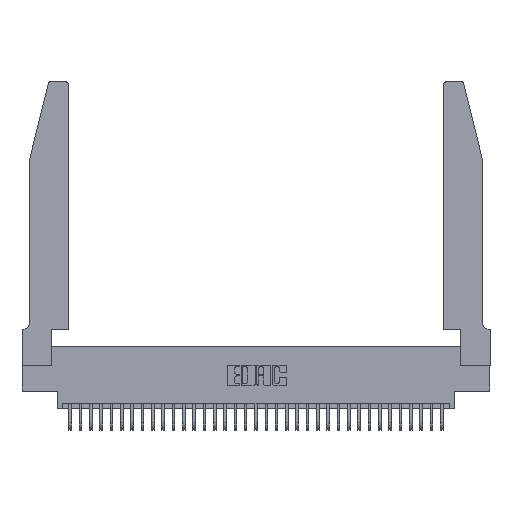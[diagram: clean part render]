
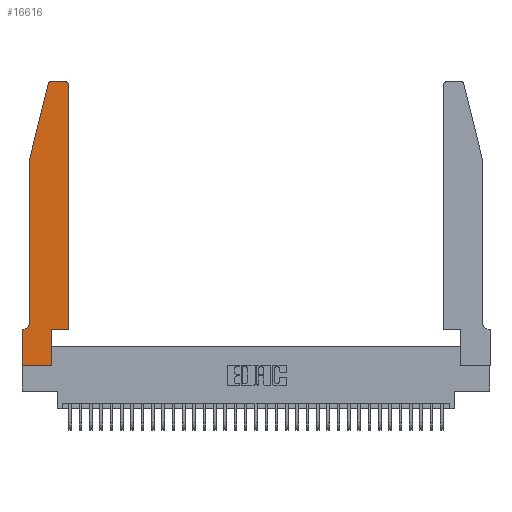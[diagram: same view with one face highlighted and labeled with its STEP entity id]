
A CAD part, top view. The second image highlights one B-rep face of the part: STEP entity #16616.
In plain terms, the highlighted planar face has unit normal (0, 0, 1).
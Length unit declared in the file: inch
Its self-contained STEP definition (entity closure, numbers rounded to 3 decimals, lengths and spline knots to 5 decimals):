
#65 = ORIENTED_EDGE ( 'NONE', *, *, #2224, .T. ) ;
#76 = VERTEX_POINT ( 'NONE', #10745 ) ;
#1164 = CARTESIAN_POINT ( 'NONE',  ( 0.4205, 2.75, 0.37 ) ) ;
#1331 = VERTEX_POINT ( 'NONE', #31870 ) ;
#1661 = VERTEX_POINT ( 'NONE', #2278 ) ;
#2116 = DIRECTION ( 'NONE',  ( -1., 0., 0. ) ) ;
#2174 = VECTOR ( 'NONE', #16784, 39.37008 ) ;
#2224 = EDGE_CURVE ( 'NONE', #10410, #76, #25357, .T. ) ;
#2278 = CARTESIAN_POINT ( 'NONE',  ( 0.2865, 0.35, 0.37 ) ) ;
#2492 = DIRECTION ( 'NONE',  ( 0., 1., 0. ) ) ;
#2646 = CARTESIAN_POINT ( 'NONE',  ( 0.4505, 2.72, 0.37 ) ) ;
#2780 = CARTESIAN_POINT ( 'NONE',  ( 0., 0., 0.37 ) ) ;
#3082 = LINE ( 'NONE', #16886, #2174 ) ;
#3813 = ORIENTED_EDGE ( 'NONE', *, *, #25505, .T. ) ;
#4161 = CARTESIAN_POINT ( 'NONE',  ( 0.0755, 2., 0.37 ) ) ;
#4770 = CARTESIAN_POINT ( 'NONE',  ( 0.0755, 2., 0.37 ) ) ;
#4788 = CARTESIAN_POINT ( 'NONE',  ( 0., 0.35, 0.37 ) ) ;
#5586 = DIRECTION ( 'NONE',  ( 1., 0., 0. ) ) ;
#5776 = EDGE_CURVE ( 'NONE', #76, #24722, #29661, .T. ) ;
#6999 = DIRECTION ( 'NONE',  ( -0.239, -0.971, 0. ) ) ;
#7488 = VERTEX_POINT ( 'NONE', #25301 ) ;
#8725 = EDGE_CURVE ( 'NONE', #26571, #1661, #8899, .T. ) ;
#8899 = LINE ( 'NONE', #36023, #22948 ) ;
#9705 = DIRECTION ( 'NONE',  ( 0., 1., 0. ) ) ;
#10109 = EDGE_CURVE ( 'NONE', #1661, #16941, #3082, .T. ) ;
#10286 = AXIS2_PLACEMENT_3D ( 'NONE', #35688, #19027, #2116 ) ;
#10410 = VERTEX_POINT ( 'NONE', #1164 ) ;
#10497 = DIRECTION ( 'NONE',  ( 0., 0., 1. ) ) ;
#10745 = CARTESIAN_POINT ( 'NONE',  ( 0.284, 2.75, 0.37 ) ) ;
#12527 = LINE ( 'NONE', #4770, #32239 ) ;
#12644 = ORIENTED_EDGE ( 'NONE', *, *, #10109, .T. ) ;
#13102 = DIRECTION ( 'NONE',  ( 0., -1., 0. ) ) ;
#13213 = ORIENTED_EDGE ( 'NONE', *, *, #24683, .T. ) ;
#13678 = CARTESIAN_POINT ( 'NONE',  ( 0.4205, 2.72, 0.37 ) ) ;
#14439 = AXIS2_PLACEMENT_3D ( 'NONE', #15244, #34764, #18112 ) ;
#15244 = CARTESIAN_POINT ( 'NONE',  ( 0.284, 2.72, 0.37 ) ) ;
#16072 = DIRECTION ( 'NONE',  ( -1., 0., 0. ) ) ;
#16124 = CARTESIAN_POINT ( 'NONE',  ( 0.0755, 0.35, 0.37 ) ) ;
#16552 = DIRECTION ( 'NONE',  ( 1., 0., 0. ) ) ;
#16616 = ADVANCED_FACE ( 'NONE', ( #25283 ), #27270, .T. ) ;
#16645 = VECTOR ( 'NONE', #5586, 39.37008 ) ;
#16696 = EDGE_CURVE ( 'NONE', #31564, #10410, #30940, .T. ) ;
#16701 = VERTEX_POINT ( 'NONE', #22013 ) ;
#16784 = DIRECTION ( 'NONE',  ( 1., 0., 0. ) ) ;
#16886 = CARTESIAN_POINT ( 'NONE',  ( 0.4505, 0.35, 0.37 ) ) ;
#16941 = VERTEX_POINT ( 'NONE', #28585 ) ;
#17128 = EDGE_CURVE ( 'NONE', #16941, #31564, #18732, .T. ) ;
#17242 = EDGE_CURVE ( 'NONE', #33891, #1331, #28287, .T. ) ;
#17891 = EDGE_CURVE ( 'NONE', #34405, #33891, #22990, .T. ) ;
#17976 = VECTOR ( 'NONE', #16072, 39.37008 ) ;
#18112 = DIRECTION ( 'NONE',  ( 1., 0., 0. ) ) ;
#18732 = LINE ( 'NONE', #26507, #31791 ) ;
#19027 = DIRECTION ( 'NONE',  ( 0., 0., -1. ) ) ;
#19042 = ORIENTED_EDGE ( 'NONE', *, *, #17128, .T. ) ;
#20008 = EDGE_CURVE ( 'NONE', #7488, #26571, #24033, .T. ) ;
#20471 = CARTESIAN_POINT ( 'NONE',  ( 0.0755, 0.42, 0.37 ) ) ;
#21068 = ORIENTED_EDGE ( 'NONE', *, *, #17242, .T. ) ;
#22013 = CARTESIAN_POINT ( 'NONE',  ( 0.0755, 2., 0.37 ) ) ;
#22519 = LINE ( 'NONE', #32684, #29059 ) ;
#22948 = VECTOR ( 'NONE', #2492, 39.37008 ) ;
#22986 = EDGE_LOOP ( 'NONE', ( #65, #32916, #13213, #27632, #23922, #21068, #3813, #27095, #24050, #12644, #19042, #27774 ) ) ;
#22990 = CIRCLE ( 'NONE', #10286, 0.07 ) ;
#23657 = CARTESIAN_POINT ( 'NONE',  ( 0.0055, 0.35, 0.37 ) ) ;
#23922 = ORIENTED_EDGE ( 'NONE', *, *, #17891, .T. ) ;
#24033 = LINE ( 'NONE', #2780, #16645 ) ;
#24050 = ORIENTED_EDGE ( 'NONE', *, *, #8725, .T. ) ;
#24683 = EDGE_CURVE ( 'NONE', #24722, #16701, #25494, .T. ) ;
#24722 = VERTEX_POINT ( 'NONE', #32375 ) ;
#25283 = FACE_OUTER_BOUND ( 'NONE', #22986, .T. ) ;
#25301 = CARTESIAN_POINT ( 'NONE',  ( 0., 0., 0.37 ) ) ;
#25357 = LINE ( 'NONE', #35562, #17976 ) ;
#25494 = LINE ( 'NONE', #4161, #32031 ) ;
#25505 = EDGE_CURVE ( 'NONE', #1331, #7488, #22519, .T. ) ;
#25740 = AXIS2_PLACEMENT_3D ( 'NONE', #4788, #10497, #30067 ) ;
#25807 = CARTESIAN_POINT ( 'NONE',  ( 0.2865, 0., 0.37 ) ) ;
#26507 = CARTESIAN_POINT ( 'NONE',  ( 0.4505, 0.35, 0.37 ) ) ;
#26571 = VERTEX_POINT ( 'NONE', #25807 ) ;
#27095 = ORIENTED_EDGE ( 'NONE', *, *, #20008, .T. ) ;
#27245 = DIRECTION ( 'NONE',  ( 0., -1., 0. ) ) ;
#27270 = PLANE ( 'NONE',  #25740 ) ;
#27632 = ORIENTED_EDGE ( 'NONE', *, *, #30723, .T. ) ;
#27774 = ORIENTED_EDGE ( 'NONE', *, *, #16696, .T. ) ;
#28287 = LINE ( 'NONE', #16124, #35681 ) ;
#28585 = CARTESIAN_POINT ( 'NONE',  ( 0.4505, 0.35, 0.37 ) ) ;
#29059 = VECTOR ( 'NONE', #13102, 39.37008 ) ;
#29661 = CIRCLE ( 'NONE', #14439, 0.03 ) ;
#30067 = DIRECTION ( 'NONE',  ( 1., 0., 0. ) ) ;
#30723 = EDGE_CURVE ( 'NONE', #16701, #34405, #12527, .T. ) ;
#30940 = CIRCLE ( 'NONE', #31347, 0.03 ) ;
#31347 = AXIS2_PLACEMENT_3D ( 'NONE', #13678, #33238, #16552 ) ;
#31564 = VERTEX_POINT ( 'NONE', #2646 ) ;
#31791 = VECTOR ( 'NONE', #9705, 39.37008 ) ;
#31870 = CARTESIAN_POINT ( 'NONE',  ( 0., 0.35, 0.37 ) ) ;
#32031 = VECTOR ( 'NONE', #6999, 39.37008 ) ;
#32239 = VECTOR ( 'NONE', #27245, 39.37008 ) ;
#32375 = CARTESIAN_POINT ( 'NONE',  ( 0.25487, 2.72718, 0.37 ) ) ;
#32684 = CARTESIAN_POINT ( 'NONE',  ( 0., 0., 0.37 ) ) ;
#32842 = DIRECTION ( 'NONE',  ( -1., 0., 0. ) ) ;
#32916 = ORIENTED_EDGE ( 'NONE', *, *, #5776, .T. ) ;
#33238 = DIRECTION ( 'NONE',  ( 0., 0., 1. ) ) ;
#33891 = VERTEX_POINT ( 'NONE', #23657 ) ;
#34405 = VERTEX_POINT ( 'NONE', #20471 ) ;
#34764 = DIRECTION ( 'NONE',  ( 0., 0., 1. ) ) ;
#35562 = CARTESIAN_POINT ( 'NONE',  ( 0.2605, 2.75, 0.37 ) ) ;
#35681 = VECTOR ( 'NONE', #32842, 39.37008 ) ;
#35688 = CARTESIAN_POINT ( 'NONE',  ( 0.0055, 0.42, 0.37 ) ) ;
#36023 = CARTESIAN_POINT ( 'NONE',  ( 0.2865, 0.35, 0.37 ) ) ;
